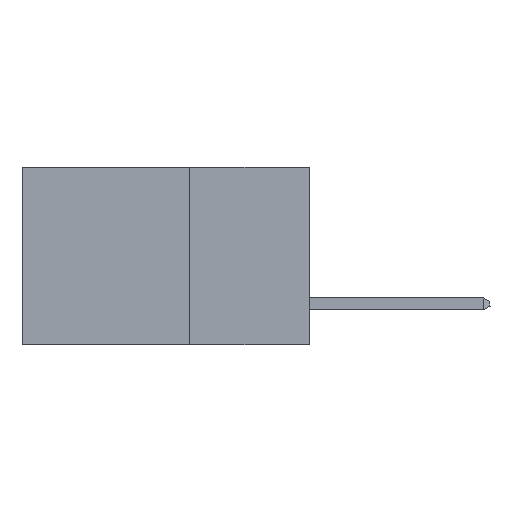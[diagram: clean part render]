
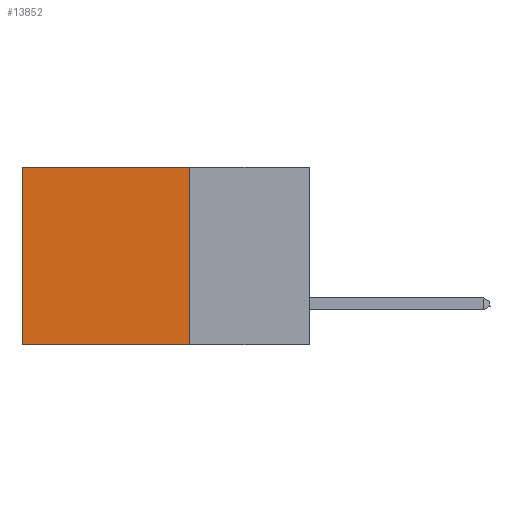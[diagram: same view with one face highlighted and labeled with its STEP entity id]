
A CAD part, left-side view. The second image highlights one B-rep face of the part: STEP entity #13852.
In plain terms, the highlighted planar face has unit normal (-1, 0, 0).
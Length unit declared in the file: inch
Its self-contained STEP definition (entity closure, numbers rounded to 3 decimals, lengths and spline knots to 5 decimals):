
#882 = LINE ( 'NONE', #7759, #10176 ) ;
#1003 = EDGE_CURVE ( 'NONE', #23937, #8175, #16332, .T. ) ;
#1240 = CARTESIAN_POINT ( 'NONE',  ( 0.2875, 0.6, -0.37 ) ) ;
#1769 = CARTESIAN_POINT ( 'NONE',  ( 0.2875, 0.25, 0. ) ) ;
#2068 = ORIENTED_EDGE ( 'NONE', *, *, #1003, .F. ) ;
#2436 = EDGE_CURVE ( 'NONE', #3814, #8175, #5753, .T. ) ;
#2527 = EDGE_LOOP ( 'NONE', ( #13905, #2068, #16978, #16684 ) ) ;
#3814 = VERTEX_POINT ( 'NONE', #8469 ) ;
#5164 = VECTOR ( 'NONE', #13595, 39.37008 ) ;
#5753 = LINE ( 'NONE', #15557, #5164 ) ;
#5972 = DIRECTION ( 'NONE',  ( 0., 0., -1. ) ) ;
#6417 = VERTEX_POINT ( 'NONE', #22684 ) ;
#7759 = CARTESIAN_POINT ( 'NONE',  ( 0.2875, 0.25, 0. ) ) ;
#8175 = VERTEX_POINT ( 'NONE', #1240 ) ;
#8459 = CARTESIAN_POINT ( 'NONE',  ( 0.2875, 0.25, 0. ) ) ;
#8469 = CARTESIAN_POINT ( 'NONE',  ( 0.2875, 0.6, 0. ) ) ;
#8926 = VECTOR ( 'NONE', #22473, 39.37008 ) ;
#10176 = VECTOR ( 'NONE', #5972, 39.37008 ) ;
#11605 = CARTESIAN_POINT ( 'NONE',  ( 0.2875, 0.25, -0.37 ) ) ;
#13595 = DIRECTION ( 'NONE',  ( 0., 0., -1. ) ) ;
#13852 = ADVANCED_FACE ( 'NONE', ( #14593 ), #14035, .F. ) ;
#13896 = LINE ( 'NONE', #1769, #8926 ) ;
#13905 = ORIENTED_EDGE ( 'NONE', *, *, #2436, .T. ) ;
#14035 = PLANE ( 'NONE',  #18819 ) ;
#14305 = VECTOR ( 'NONE', #22956, 39.37008 ) ;
#14545 = CARTESIAN_POINT ( 'NONE',  ( 0.2875, 0.25, -0.37 ) ) ;
#14593 = FACE_OUTER_BOUND ( 'NONE', #2527, .T. ) ;
#15557 = CARTESIAN_POINT ( 'NONE',  ( 0.2875, 0.6, 0. ) ) ;
#16332 = LINE ( 'NONE', #11605, #14305 ) ;
#16684 = ORIENTED_EDGE ( 'NONE', *, *, #16691, .T. ) ;
#16691 = EDGE_CURVE ( 'NONE', #6417, #3814, #13896, .T. ) ;
#16978 = ORIENTED_EDGE ( 'NONE', *, *, #24142, .F. ) ;
#18819 = AXIS2_PLACEMENT_3D ( 'NONE', #8459, #19842, #23500 ) ;
#19842 = DIRECTION ( 'NONE',  ( 1., 0., 0. ) ) ;
#22473 = DIRECTION ( 'NONE',  ( 0., 1., 0. ) ) ;
#22684 = CARTESIAN_POINT ( 'NONE',  ( 0.2875, 0.25, 0. ) ) ;
#22956 = DIRECTION ( 'NONE',  ( 0., 1., 0. ) ) ;
#23500 = DIRECTION ( 'NONE',  ( 0., 0., -1. ) ) ;
#23937 = VERTEX_POINT ( 'NONE', #14545 ) ;
#24142 = EDGE_CURVE ( 'NONE', #6417, #23937, #882, .T. ) ;
